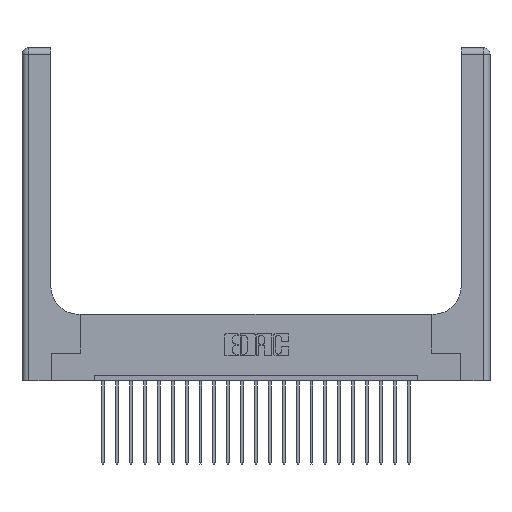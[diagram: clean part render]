
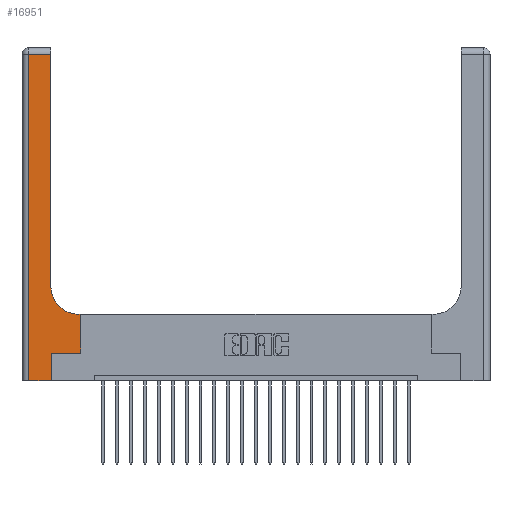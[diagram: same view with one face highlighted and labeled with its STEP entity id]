
A CAD part, top view. The second image highlights one B-rep face of the part: STEP entity #16951.
In plain terms, the highlighted planar face has unit normal (0, 0, 1).
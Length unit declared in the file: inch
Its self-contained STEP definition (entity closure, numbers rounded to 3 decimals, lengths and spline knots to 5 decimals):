
#187 = CIRCLE ( 'NONE', #16352, 0.25 ) ;
#448 = AXIS2_PLACEMENT_3D ( 'NONE', #17849, #4336, #6079 ) ;
#466 = EDGE_CURVE ( 'NONE', #15727, #14563, #2101, .T. ) ;
#542 = VECTOR ( 'NONE', #14669, 39.37008 ) ;
#636 = EDGE_CURVE ( 'NONE', #15270, #18968, #13912, .T. ) ;
#808 = CARTESIAN_POINT ( 'NONE',  ( 0.528, 0.25, 0.37 ) ) ;
#881 = DIRECTION ( 'NONE',  ( 0., 1., 0. ) ) ;
#1064 = LINE ( 'NONE', #2671, #542 ) ;
#1159 = VECTOR ( 'NONE', #881, 39.37008 ) ;
#1620 = DIRECTION ( 'NONE',  ( -1., 0., 0. ) ) ;
#1775 = CARTESIAN_POINT ( 'NONE',  ( 0.265, 0.25, 0.37 ) ) ;
#1846 = CARTESIAN_POINT ( 'NONE',  ( 0., 2.94, 0.37 ) ) ;
#2101 = LINE ( 'NONE', #13256, #5910 ) ;
#2343 = VECTOR ( 'NONE', #18886, 39.37008 ) ;
#2374 = ORIENTED_EDGE ( 'NONE', *, *, #636, .T. ) ;
#2427 = DIRECTION ( 'NONE',  ( 0., -1., 0. ) ) ;
#2428 = PLANE ( 'NONE',  #448 ) ;
#2671 = CARTESIAN_POINT ( 'NONE',  ( 0., 0., 0.37 ) ) ;
#2925 = CARTESIAN_POINT ( 'NONE',  ( 0.528, 0.6, 0.37 ) ) ;
#3110 = DIRECTION ( 'NONE',  ( 0., 1., 0. ) ) ;
#3578 = VERTEX_POINT ( 'NONE', #2925 ) ;
#3653 = CARTESIAN_POINT ( 'NONE',  ( 0.265, 0.25, 0.37 ) ) ;
#4336 = DIRECTION ( 'NONE',  ( 0., 0., -1. ) ) ;
#4531 = EDGE_CURVE ( 'NONE', #12235, #10586, #12614, .T. ) ;
#4567 = ORIENTED_EDGE ( 'NONE', *, *, #9444, .T. ) ;
#4658 = ORIENTED_EDGE ( 'NONE', *, *, #16429, .T. ) ;
#4977 = CARTESIAN_POINT ( 'NONE',  ( 0.51, 0.85, 0.37 ) ) ;
#5152 = CARTESIAN_POINT ( 'NONE',  ( 0.26, 3., 0.37 ) ) ;
#5481 = EDGE_CURVE ( 'NONE', #14563, #15312, #22055, .T. ) ;
#5644 = ORIENTED_EDGE ( 'NONE', *, *, #18279, .T. ) ;
#5910 = VECTOR ( 'NONE', #3110, 39.37008 ) ;
#6079 = DIRECTION ( 'NONE',  ( -1., 0., 0. ) ) ;
#6379 = VERTEX_POINT ( 'NONE', #13355 ) ;
#6572 = ORIENTED_EDGE ( 'NONE', *, *, #4531, .T. ) ;
#6729 = DIRECTION ( 'NONE',  ( 0., 0., -1. ) ) ;
#7539 = EDGE_CURVE ( 'NONE', #6379, #15270, #187, .T. ) ;
#9102 = ORIENTED_EDGE ( 'NONE', *, *, #15865, .T. ) ;
#9183 = CARTESIAN_POINT ( 'NONE',  ( 0.265, 0., 0.37 ) ) ;
#9444 = EDGE_CURVE ( 'NONE', #15312, #3578, #10552, .T. ) ;
#10134 = LINE ( 'NONE', #11420, #20187 ) ;
#10148 = DIRECTION ( 'NONE',  ( 1., 0., 0. ) ) ;
#10552 = LINE ( 'NONE', #808, #1159 ) ;
#10586 = VERTEX_POINT ( 'NONE', #14916 ) ;
#10633 = ORIENTED_EDGE ( 'NONE', *, *, #5481, .T. ) ;
#11062 = FACE_OUTER_BOUND ( 'NONE', #15501, .T. ) ;
#11420 = CARTESIAN_POINT ( 'NONE',  ( 0.26, 0.6, 0.37 ) ) ;
#11594 = ORIENTED_EDGE ( 'NONE', *, *, #466, .T. ) ;
#12235 = VERTEX_POINT ( 'NONE', #15687 ) ;
#12334 = VECTOR ( 'NONE', #17030, 39.37008 ) ;
#12614 = LINE ( 'NONE', #16257, #15764 ) ;
#13213 = LINE ( 'NONE', #1846, #15311 ) ;
#13256 = CARTESIAN_POINT ( 'NONE',  ( 0.265, 0., 0.37 ) ) ;
#13355 = CARTESIAN_POINT ( 'NONE',  ( 0.51, 0.6, 0.37 ) ) ;
#13912 = LINE ( 'NONE', #5152, #12334 ) ;
#14563 = VERTEX_POINT ( 'NONE', #3653 ) ;
#14613 = CARTESIAN_POINT ( 'NONE',  ( 0.26, 2.94, 0.37 ) ) ;
#14669 = DIRECTION ( 'NONE',  ( 1., 0., 0. ) ) ;
#14916 = CARTESIAN_POINT ( 'NONE',  ( 0.06, 0., 0.37 ) ) ;
#15270 = VERTEX_POINT ( 'NONE', #21905 ) ;
#15311 = VECTOR ( 'NONE', #1620, 39.37008 ) ;
#15312 = VERTEX_POINT ( 'NONE', #16668 ) ;
#15501 = EDGE_LOOP ( 'NONE', ( #2374, #9102, #6572, #5644, #11594, #10633, #4567, #4658, #18457 ) ) ;
#15687 = CARTESIAN_POINT ( 'NONE',  ( 0.06, 2.94, 0.37 ) ) ;
#15727 = VERTEX_POINT ( 'NONE', #9183 ) ;
#15764 = VECTOR ( 'NONE', #2427, 39.37008 ) ;
#15865 = EDGE_CURVE ( 'NONE', #18968, #12235, #13213, .T. ) ;
#16257 = CARTESIAN_POINT ( 'NONE',  ( 0.06, 3., 0.37 ) ) ;
#16352 = AXIS2_PLACEMENT_3D ( 'NONE', #4977, #6729, #10148 ) ;
#16429 = EDGE_CURVE ( 'NONE', #3578, #6379, #10134, .T. ) ;
#16668 = CARTESIAN_POINT ( 'NONE',  ( 0.528, 0.25, 0.37 ) ) ;
#16951 = ADVANCED_FACE ( 'NONE', ( #11062 ), #2428, .F. ) ;
#17030 = DIRECTION ( 'NONE',  ( 0., 1., 0. ) ) ;
#17849 = CARTESIAN_POINT ( 'NONE',  ( 0., 3., 0.37 ) ) ;
#17945 = DIRECTION ( 'NONE',  ( -1., 0., 0. ) ) ;
#18279 = EDGE_CURVE ( 'NONE', #10586, #15727, #1064, .T. ) ;
#18457 = ORIENTED_EDGE ( 'NONE', *, *, #7539, .T. ) ;
#18886 = DIRECTION ( 'NONE',  ( 1., 0., 0. ) ) ;
#18968 = VERTEX_POINT ( 'NONE', #14613 ) ;
#20187 = VECTOR ( 'NONE', #17945, 39.37008 ) ;
#21905 = CARTESIAN_POINT ( 'NONE',  ( 0.26, 0.85, 0.37 ) ) ;
#22055 = LINE ( 'NONE', #1775, #2343 ) ;
